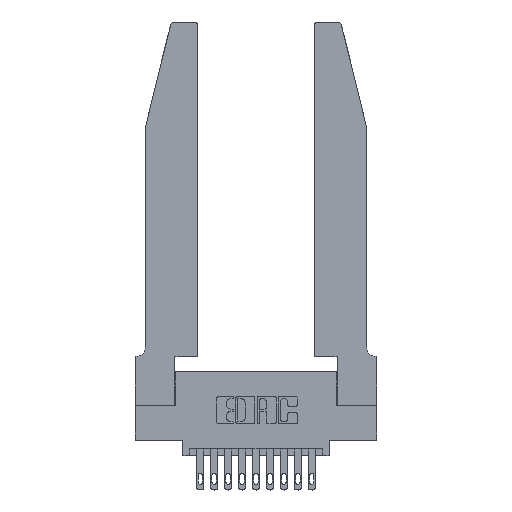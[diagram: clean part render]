
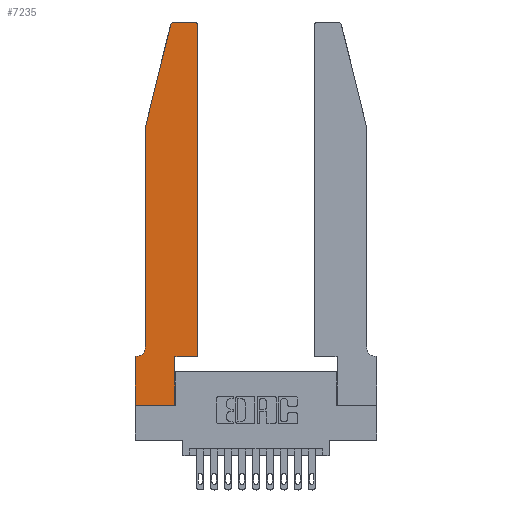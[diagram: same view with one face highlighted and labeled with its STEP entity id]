
A CAD part, top view. The second image highlights one B-rep face of the part: STEP entity #7235.
In plain terms, the highlighted planar face has unit normal (0, 0, 1).
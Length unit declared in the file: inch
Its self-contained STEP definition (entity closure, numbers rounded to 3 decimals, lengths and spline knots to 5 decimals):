
#675 = ORIENTED_EDGE ( 'NONE', *, *, #1804, .T. ) ;
#742 = ORIENTED_EDGE ( 'NONE', *, *, #3384, .T. ) ;
#953 = EDGE_CURVE ( 'NONE', #10324, #7364, #10441, .T. ) ;
#1038 = EDGE_LOOP ( 'NONE', ( #4976, #7670, #9536, #12706, #1573, #742, #2369, #14156, #11908, #10004, #675, #8518 ) ) ;
#1323 = CARTESIAN_POINT ( 'NONE',  ( 0.2865, 0.35, 0.37 ) ) ;
#1573 = ORIENTED_EDGE ( 'NONE', *, *, #12100, .T. ) ;
#1679 = CARTESIAN_POINT ( 'NONE',  ( 0.2865, 0., 0.37 ) ) ;
#1804 = EDGE_CURVE ( 'NONE', #7364, #15134, #12573, .T. ) ;
#2059 = CARTESIAN_POINT ( 'NONE',  ( 0.4505, 2.72, 0.37 ) ) ;
#2277 = VERTEX_POINT ( 'NONE', #7190 ) ;
#2364 = CARTESIAN_POINT ( 'NONE',  ( 0.4505, 0.35, 0.37 ) ) ;
#2369 = ORIENTED_EDGE ( 'NONE', *, *, #11975, .T. ) ;
#2940 = CARTESIAN_POINT ( 'NONE',  ( 0., 0.35, 0.37 ) ) ;
#3383 = CARTESIAN_POINT ( 'NONE',  ( 0.0755, 0.35, 0.37 ) ) ;
#3384 = EDGE_CURVE ( 'NONE', #15850, #13517, #8432, .T. ) ;
#3454 = DIRECTION ( 'NONE',  ( -0.239, -0.971, 0. ) ) ;
#3668 = CARTESIAN_POINT ( 'NONE',  ( 0.4505, 0.35, 0.37 ) ) ;
#3695 = DIRECTION ( 'NONE',  ( 0., 1., 0. ) ) ;
#3719 = VECTOR ( 'NONE', #6158, 39.37008 ) ;
#3912 = CARTESIAN_POINT ( 'NONE',  ( 0.0055, 0.42, 0.37 ) ) ;
#4006 = AXIS2_PLACEMENT_3D ( 'NONE', #4278, #15794, #13074 ) ;
#4278 = CARTESIAN_POINT ( 'NONE',  ( 0.284, 2.72, 0.37 ) ) ;
#4281 = DIRECTION ( 'NONE',  ( 0., -1., 0. ) ) ;
#4324 = EDGE_CURVE ( 'NONE', #11747, #11167, #6393, .T. ) ;
#4398 = VERTEX_POINT ( 'NONE', #5546 ) ;
#4538 = LINE ( 'NONE', #13427, #9690 ) ;
#4676 = CARTESIAN_POINT ( 'NONE',  ( 0.284, 2.75, 0.37 ) ) ;
#4924 = DIRECTION ( 'NONE',  ( 1., 0., 0. ) ) ;
#4976 = ORIENTED_EDGE ( 'NONE', *, *, #7118, .T. ) ;
#5546 = CARTESIAN_POINT ( 'NONE',  ( 0.0755, 2., 0.37 ) ) ;
#5870 = DIRECTION ( 'NONE',  ( 1., 0., 0. ) ) ;
#5935 = CARTESIAN_POINT ( 'NONE',  ( 0.0755, 0.42, 0.37 ) ) ;
#5941 = AXIS2_PLACEMENT_3D ( 'NONE', #6924, #15815, #12011 ) ;
#5951 = VERTEX_POINT ( 'NONE', #1679 ) ;
#6108 = CARTESIAN_POINT ( 'NONE',  ( 0., 0., 0.37 ) ) ;
#6151 = CARTESIAN_POINT ( 'NONE',  ( 0.0055, 0.35, 0.37 ) ) ;
#6158 = DIRECTION ( 'NONE',  ( 0., -1., 0. ) ) ;
#6393 = CIRCLE ( 'NONE', #4006, 0.03 ) ;
#6496 = EDGE_CURVE ( 'NONE', #4398, #13808, #15224, .T. ) ;
#6681 = PLANE ( 'NONE',  #8721 ) ;
#6905 = VECTOR ( 'NONE', #4281, 39.37008 ) ;
#6924 = CARTESIAN_POINT ( 'NONE',  ( 0.4205, 2.72, 0.37 ) ) ;
#6992 = CARTESIAN_POINT ( 'NONE',  ( 0., 0., 0.37 ) ) ;
#7118 = EDGE_CURVE ( 'NONE', #2277, #11747, #13848, .T. ) ;
#7190 = CARTESIAN_POINT ( 'NONE',  ( 0.4205, 2.75, 0.37 ) ) ;
#7235 = ADVANCED_FACE ( 'NONE', ( #11654 ), #6681, .T. ) ;
#7357 = CARTESIAN_POINT ( 'NONE',  ( 0.0755, 2., 0.37 ) ) ;
#7364 = VERTEX_POINT ( 'NONE', #15262 ) ;
#7505 = VECTOR ( 'NONE', #10795, 39.37008 ) ;
#7670 = ORIENTED_EDGE ( 'NONE', *, *, #4324, .T. ) ;
#8116 = EDGE_CURVE ( 'NONE', #8703, #5951, #4538, .T. ) ;
#8141 = CARTESIAN_POINT ( 'NONE',  ( 0.2605, 2.75, 0.37 ) ) ;
#8432 = LINE ( 'NONE', #3383, #15910 ) ;
#8518 = ORIENTED_EDGE ( 'NONE', *, *, #9226, .T. ) ;
#8703 = VERTEX_POINT ( 'NONE', #6992 ) ;
#8721 = AXIS2_PLACEMENT_3D ( 'NONE', #2940, #13057, #11764 ) ;
#9226 = EDGE_CURVE ( 'NONE', #15134, #2277, #10631, .T. ) ;
#9536 = ORIENTED_EDGE ( 'NONE', *, *, #10756, .T. ) ;
#9563 = CARTESIAN_POINT ( 'NONE',  ( 0.2865, 0.35, 0.37 ) ) ;
#9690 = VECTOR ( 'NONE', #5870, 39.37008 ) ;
#10004 = ORIENTED_EDGE ( 'NONE', *, *, #953, .T. ) ;
#10233 = AXIS2_PLACEMENT_3D ( 'NONE', #3912, #12671, #13945 ) ;
#10324 = VERTEX_POINT ( 'NONE', #9563 ) ;
#10441 = LINE ( 'NONE', #3668, #14753 ) ;
#10631 = CIRCLE ( 'NONE', #5941, 0.03 ) ;
#10756 = EDGE_CURVE ( 'NONE', #11167, #4398, #12428, .T. ) ;
#10795 = DIRECTION ( 'NONE',  ( -1., 0., 0. ) ) ;
#11167 = VERTEX_POINT ( 'NONE', #14548 ) ;
#11654 = FACE_OUTER_BOUND ( 'NONE', #1038, .T. ) ;
#11747 = VERTEX_POINT ( 'NONE', #4676 ) ;
#11764 = DIRECTION ( 'NONE',  ( 1., 0., 0. ) ) ;
#11908 = ORIENTED_EDGE ( 'NONE', *, *, #16050, .T. ) ;
#11975 = EDGE_CURVE ( 'NONE', #13517, #8703, #14351, .T. ) ;
#12011 = DIRECTION ( 'NONE',  ( 1., 0., 0. ) ) ;
#12100 = EDGE_CURVE ( 'NONE', #13808, #15850, #12948, .T. ) ;
#12428 = LINE ( 'NONE', #7357, #16198 ) ;
#12573 = LINE ( 'NONE', #2364, #14332 ) ;
#12605 = DIRECTION ( 'NONE',  ( 0., 1., 0. ) ) ;
#12671 = DIRECTION ( 'NONE',  ( 0., 0., -1. ) ) ;
#12706 = ORIENTED_EDGE ( 'NONE', *, *, #6496, .T. ) ;
#12948 = CIRCLE ( 'NONE', #10233, 0.07 ) ;
#13057 = DIRECTION ( 'NONE',  ( 0., 0., 1. ) ) ;
#13074 = DIRECTION ( 'NONE',  ( 1., 0., 0. ) ) ;
#13427 = CARTESIAN_POINT ( 'NONE',  ( 0., 0., 0.37 ) ) ;
#13498 = DIRECTION ( 'NONE',  ( -1., 0., 0. ) ) ;
#13517 = VERTEX_POINT ( 'NONE', #15670 ) ;
#13808 = VERTEX_POINT ( 'NONE', #5935 ) ;
#13848 = LINE ( 'NONE', #8141, #7505 ) ;
#13945 = DIRECTION ( 'NONE',  ( -1., 0., 0. ) ) ;
#14156 = ORIENTED_EDGE ( 'NONE', *, *, #8116, .T. ) ;
#14250 = VECTOR ( 'NONE', #3695, 39.37008 ) ;
#14332 = VECTOR ( 'NONE', #12605, 39.37008 ) ;
#14351 = LINE ( 'NONE', #6108, #3719 ) ;
#14548 = CARTESIAN_POINT ( 'NONE',  ( 0.25487, 2.72718, 0.37 ) ) ;
#14753 = VECTOR ( 'NONE', #4924, 39.37008 ) ;
#15134 = VERTEX_POINT ( 'NONE', #2059 ) ;
#15224 = LINE ( 'NONE', #15676, #6905 ) ;
#15262 = CARTESIAN_POINT ( 'NONE',  ( 0.4505, 0.35, 0.37 ) ) ;
#15615 = LINE ( 'NONE', #1323, #14250 ) ;
#15670 = CARTESIAN_POINT ( 'NONE',  ( 0., 0.35, 0.37 ) ) ;
#15676 = CARTESIAN_POINT ( 'NONE',  ( 0.0755, 2., 0.37 ) ) ;
#15794 = DIRECTION ( 'NONE',  ( 0., 0., 1. ) ) ;
#15815 = DIRECTION ( 'NONE',  ( 0., 0., 1. ) ) ;
#15850 = VERTEX_POINT ( 'NONE', #6151 ) ;
#15910 = VECTOR ( 'NONE', #13498, 39.37008 ) ;
#16050 = EDGE_CURVE ( 'NONE', #5951, #10324, #15615, .T. ) ;
#16198 = VECTOR ( 'NONE', #3454, 39.37008 ) ;
